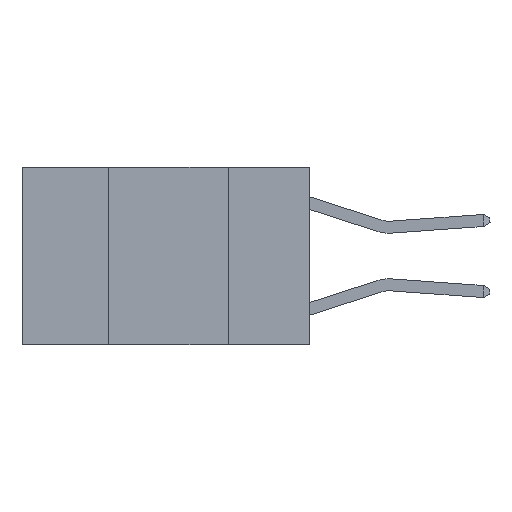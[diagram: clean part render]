
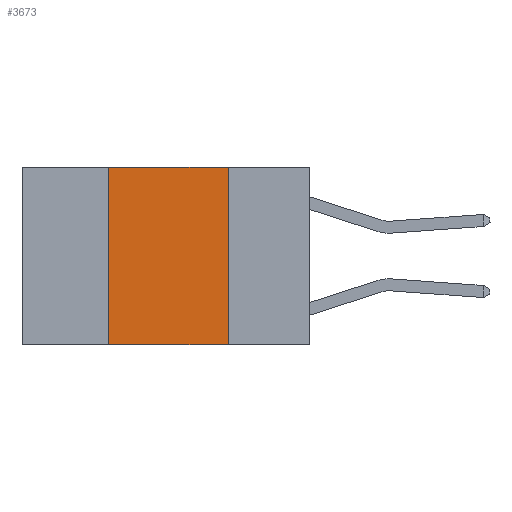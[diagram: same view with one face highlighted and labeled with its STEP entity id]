
A CAD part, left-side view. The second image highlights one B-rep face of the part: STEP entity #3673.
In plain terms, the highlighted planar face has unit normal (-1, 0, 0).
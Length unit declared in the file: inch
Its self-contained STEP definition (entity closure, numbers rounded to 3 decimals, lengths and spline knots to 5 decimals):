
#582 = CARTESIAN_POINT ( 'NONE',  ( 0., 0.6, -0.37 ) ) ;
#941 = DIRECTION ( 'NONE',  ( 0., 0., -1. ) ) ;
#1396 = EDGE_LOOP ( 'NONE', ( #6568, #6584, #6664, #6692 ) ) ;
#1502 = CARTESIAN_POINT ( 'NONE',  ( 0., 0.42, 0. ) ) ;
#1628 = EDGE_CURVE ( 'NONE', #8678, #3027, #7282, .T. ) ;
#1638 = VECTOR ( 'NONE', #6821, 39.37008 ) ;
#1906 = EDGE_CURVE ( 'NONE', #3027, #4709, #7756, .T. ) ;
#2098 = DIRECTION ( 'NONE',  ( 0., -1., 0. ) ) ;
#2231 = CARTESIAN_POINT ( 'NONE',  ( 0., 0.17, -0.37 ) ) ;
#2454 = DIRECTION ( 'NONE',  ( 0., -1., 0. ) ) ;
#3027 = VERTEX_POINT ( 'NONE', #8603 ) ;
#3673 = ADVANCED_FACE ( 'NONE', ( #6896 ), #7283, .F. ) ;
#3902 = DIRECTION ( 'NONE',  ( 0., 0., -1. ) ) ;
#4709 = VERTEX_POINT ( 'NONE', #5945 ) ;
#4898 = VECTOR ( 'NONE', #2454, 39.37008 ) ;
#5241 = CARTESIAN_POINT ( 'NONE',  ( 0., 0.6, 0. ) ) ;
#5401 = AXIS2_PLACEMENT_3D ( 'NONE', #9191, #7889, #3902 ) ;
#5945 = CARTESIAN_POINT ( 'NONE',  ( 0., 0.17, 0. ) ) ;
#6568 = ORIENTED_EDGE ( 'NONE', *, *, #7457, .F. ) ;
#6584 = ORIENTED_EDGE ( 'NONE', *, *, #1906, .F. ) ;
#6664 = ORIENTED_EDGE ( 'NONE', *, *, #1628, .F. ) ;
#6667 = LINE ( 'NONE', #582, #4898 ) ;
#6692 = ORIENTED_EDGE ( 'NONE', *, *, #6860, .T. ) ;
#6821 = DIRECTION ( 'NONE',  ( 0., 0., 1. ) ) ;
#6860 = EDGE_CURVE ( 'NONE', #8678, #8327, #6667, .T. ) ;
#6896 = FACE_OUTER_BOUND ( 'NONE', #1396, .T. ) ;
#7282 = LINE ( 'NONE', #1502, #1638 ) ;
#7283 = PLANE ( 'NONE',  #5401 ) ;
#7457 = EDGE_CURVE ( 'NONE', #4709, #8327, #8494, .T. ) ;
#7573 = VECTOR ( 'NONE', #2098, 39.37008 ) ;
#7756 = LINE ( 'NONE', #5241, #7573 ) ;
#7889 = DIRECTION ( 'NONE',  ( 1., 0., 0. ) ) ;
#8253 = CARTESIAN_POINT ( 'NONE',  ( 0., 0.17, 0. ) ) ;
#8286 = VECTOR ( 'NONE', #941, 39.37008 ) ;
#8327 = VERTEX_POINT ( 'NONE', #2231 ) ;
#8494 = LINE ( 'NONE', #8253, #8286 ) ;
#8603 = CARTESIAN_POINT ( 'NONE',  ( 0., 0.42, 0. ) ) ;
#8678 = VERTEX_POINT ( 'NONE', #9308 ) ;
#9191 = CARTESIAN_POINT ( 'NONE',  ( 0., 0.6, 0. ) ) ;
#9308 = CARTESIAN_POINT ( 'NONE',  ( 0., 0.42, -0.37 ) ) ;
